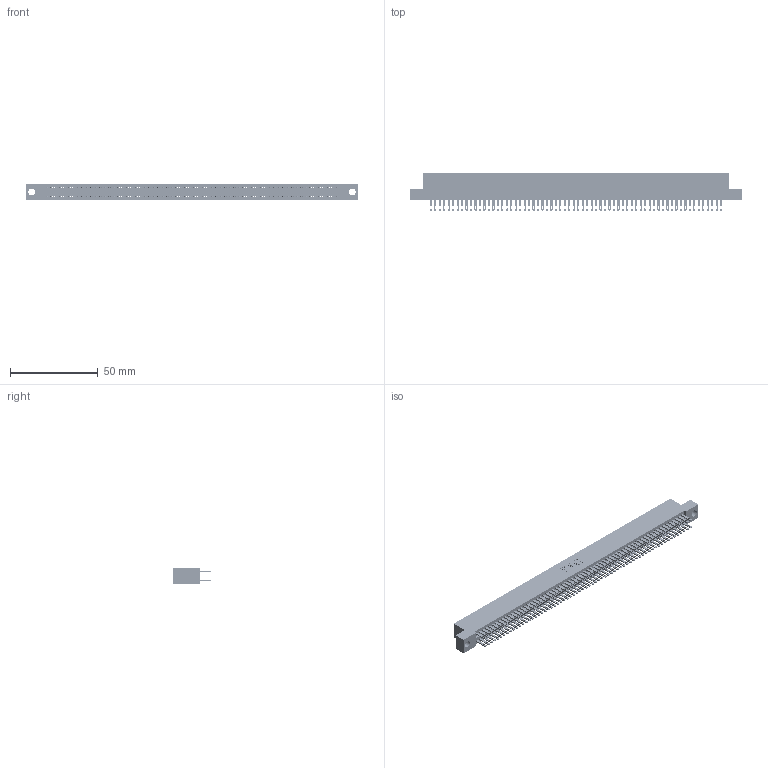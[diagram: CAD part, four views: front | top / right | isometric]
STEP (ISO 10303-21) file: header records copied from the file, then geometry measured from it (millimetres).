
FILE_DESCRIPTION (( 'STEP AP203' ), '1' );
FILE_NAME ('345-132-500-204.STEP', '2018-10-20T02:51:49', ( '' ), ( '' ), 'SwSTEP 2.0', 'SolidWorks 2016', '' );
FILE_SCHEMA (( 'CONFIG_CONTROL_DESIGN' ));
Length unit declared in the file: inch
Products named in the file (3): 345 Part_Flush Mounting Lugs - 0.156 Dia-TH; 345-292-001_345-293-100; 345-132-500-204
Assembly tree (133 placements, depth 2):
  345-132-500-204
    345 Part_Flush Mounting Lugs - 0.156 Dia-TH
    345-292-001_345-293-100  x132
Bounding box: 188.85 x 21.51 x 9.4 mm (x, y, z)
Volume: 18883.3 mm3; surface area: 29539 mm2
Topology: 133 solids, 133 shells, 6198 faces, 18953 edges, 12634 vertices
Faces by surface type: plane 3644, cylinder 2554
Entity records: 48487 total; most frequent: CARTESIAN_POINT 8104, ORIENTED_EDGE 8038, DIRECTION 7119, EDGE_CURVE 4019, LINE 3619, VECTOR 3619, VERTEX_POINT 2678, AXIS2_PLACEMENT_3D 1750
